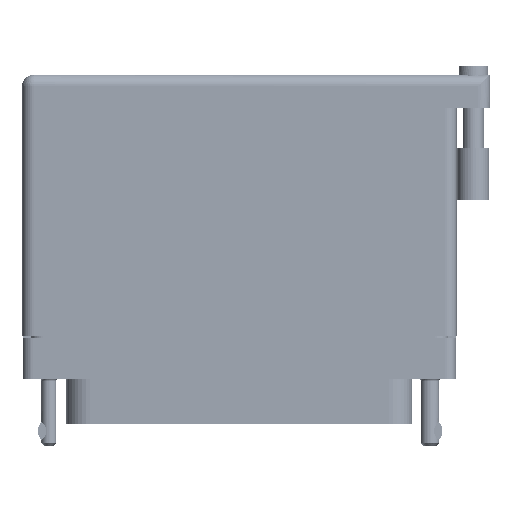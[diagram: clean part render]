
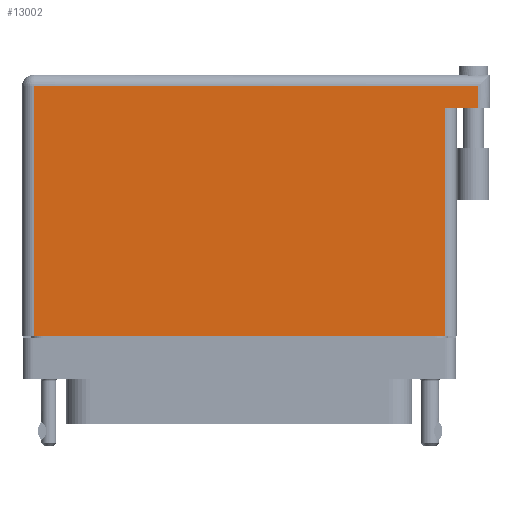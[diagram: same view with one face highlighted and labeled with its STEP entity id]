
A CAD part, front view. The second image highlights one B-rep face of the part: STEP entity #13002.
In plain terms, the highlighted face is planar.
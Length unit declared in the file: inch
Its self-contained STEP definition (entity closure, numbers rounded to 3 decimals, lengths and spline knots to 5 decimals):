
#2901 = EDGE_LOOP ( 'NONE', ( #37580, #12818, #54215, #3720, #56493, #22698 ) ) ;
#3175 = DIRECTION ( 'NONE',  ( -1., 0., 0. ) ) ;
#3720 = ORIENTED_EDGE ( 'NONE', *, *, #48558, .T. ) ;
#4200 = CARTESIAN_POINT ( 'NONE',  ( 1.5, 1.269, 0.4495 ) ) ;
#4644 = CARTESIAN_POINT ( 'NONE',  ( -1.3, 1.396, 0.4495 ) ) ;
#7366 = VECTOR ( 'NONE', #9364, 39.37008 ) ;
#9364 = DIRECTION ( 'NONE',  ( -1., 0., 0. ) ) ;
#12818 = ORIENTED_EDGE ( 'NONE', *, *, #20820, .T. ) ;
#12953 = LINE ( 'NONE', #26798, #34264 ) ;
#12988 = CARTESIAN_POINT ( 'NONE',  ( 1.23, 1.269, 0.4495 ) ) ;
#13002 = ADVANCED_FACE ( 'NONE', ( #25513 ), #26561, .F. ) ;
#14806 = VERTEX_POINT ( 'NONE', #52904 ) ;
#15120 = VECTOR ( 'NONE', #18177, 39.37008 ) ;
#18177 = DIRECTION ( 'NONE',  ( -1., 0., 0. ) ) ;
#19440 = DIRECTION ( 'NONE',  ( 0., 1., 0. ) ) ;
#20362 = EDGE_CURVE ( 'NONE', #36233, #23034, #12953, .T. ) ;
#20820 = EDGE_CURVE ( 'NONE', #23034, #25677, #56258, .T. ) ;
#22209 = DIRECTION ( 'NONE',  ( 0., 1., 0. ) ) ;
#22698 = ORIENTED_EDGE ( 'NONE', *, *, #32351, .T. ) ;
#23034 = VERTEX_POINT ( 'NONE', #28367 ) ;
#25513 = FACE_OUTER_BOUND ( 'NONE', #2901, .T. ) ;
#25677 = VERTEX_POINT ( 'NONE', #60678 ) ;
#26561 = PLANE ( 'NONE',  #31073 ) ;
#26798 = CARTESIAN_POINT ( 'NONE',  ( -1.3, -0.1, 0.4495 ) ) ;
#28326 = EDGE_CURVE ( 'NONE', #14806, #45658, #40121, .T. ) ;
#28367 = CARTESIAN_POINT ( 'NONE',  ( 1.23, -0.1, 0.4495 ) ) ;
#29268 = CARTESIAN_POINT ( 'NONE',  ( 1.43, 1.466, 0.4495 ) ) ;
#30991 = LINE ( 'NONE', #31282, #41312 ) ;
#31073 = AXIS2_PLACEMENT_3D ( 'NONE', #59457, #31236, #3175 ) ;
#31236 = DIRECTION ( 'NONE',  ( 0., 0., -1. ) ) ;
#31282 = CARTESIAN_POINT ( 'NONE',  ( -1.23, -0.1, 0.4495 ) ) ;
#32351 = EDGE_CURVE ( 'NONE', #45658, #36233, #30991, .T. ) ;
#34264 = VECTOR ( 'NONE', #45295, 39.37008 ) ;
#36233 = VERTEX_POINT ( 'NONE', #53007 ) ;
#36920 = EDGE_CURVE ( 'NONE', #53592, #25677, #45529, .T. ) ;
#37580 = ORIENTED_EDGE ( 'NONE', *, *, #20362, .T. ) ;
#39291 = LINE ( 'NONE', #29268, #51002 ) ;
#40121 = LINE ( 'NONE', #4644, #15120 ) ;
#41312 = VECTOR ( 'NONE', #59311, 39.37008 ) ;
#45295 = DIRECTION ( 'NONE',  ( 1., 0., 0. ) ) ;
#45529 = LINE ( 'NONE', #4200, #7366 ) ;
#45658 = VERTEX_POINT ( 'NONE', #53191 ) ;
#48558 = EDGE_CURVE ( 'NONE', #53592, #14806, #39291, .T. ) ;
#48922 = VECTOR ( 'NONE', #22209, 39.37008 ) ;
#51002 = VECTOR ( 'NONE', #19440, 39.37008 ) ;
#52904 = CARTESIAN_POINT ( 'NONE',  ( 1.43, 1.396, 0.4495 ) ) ;
#53007 = CARTESIAN_POINT ( 'NONE',  ( -1.23, -0.1, 0.4495 ) ) ;
#53191 = CARTESIAN_POINT ( 'NONE',  ( -1.23, 1.396, 0.4495 ) ) ;
#53592 = VERTEX_POINT ( 'NONE', #56817 ) ;
#54215 = ORIENTED_EDGE ( 'NONE', *, *, #36920, .F. ) ;
#56258 = LINE ( 'NONE', #12988, #48922 ) ;
#56493 = ORIENTED_EDGE ( 'NONE', *, *, #28326, .T. ) ;
#56817 = CARTESIAN_POINT ( 'NONE',  ( 1.43, 1.269, 0.4495 ) ) ;
#59311 = DIRECTION ( 'NONE',  ( 0., -1., 0. ) ) ;
#59457 = CARTESIAN_POINT ( 'NONE',  ( -1.3, 1.466, 0.4495 ) ) ;
#60678 = CARTESIAN_POINT ( 'NONE',  ( 1.23, 1.269, 0.4495 ) ) ;
